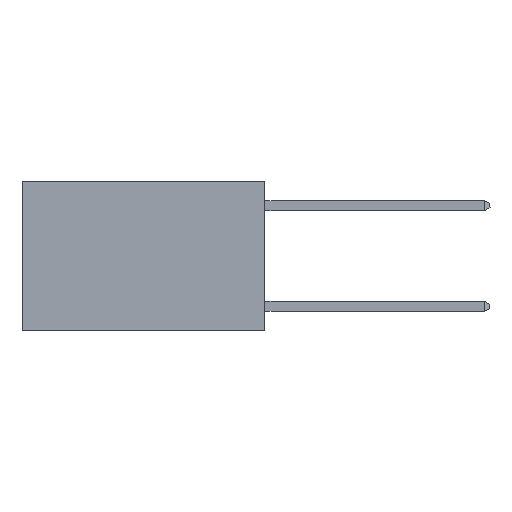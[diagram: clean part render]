
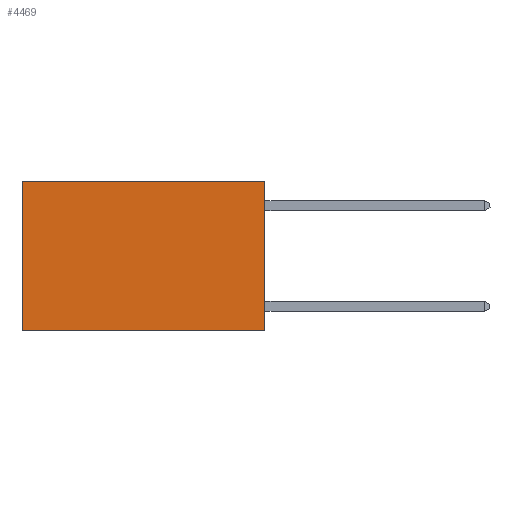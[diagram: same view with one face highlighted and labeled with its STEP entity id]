
A CAD part, left-side view. The second image highlights one B-rep face of the part: STEP entity #4469.
In plain terms, the highlighted planar face has unit normal (-1, 0, 0).
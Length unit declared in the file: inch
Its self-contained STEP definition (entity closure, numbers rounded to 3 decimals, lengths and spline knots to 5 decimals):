
#91 = FACE_OUTER_BOUND ( 'NONE', #1122, .T. ) ;
#298 = CARTESIAN_POINT ( 'NONE',  ( 0.2625, 0., 0. ) ) ;
#379 = EDGE_CURVE ( 'NONE', #6672, #7681, #6910, .T. ) ;
#523 = LINE ( 'NONE', #5374, #2490 ) ;
#844 = CARTESIAN_POINT ( 'NONE',  ( 0.2625, 0.6, -0.37 ) ) ;
#884 = PLANE ( 'NONE',  #6083 ) ;
#1122 = EDGE_LOOP ( 'NONE', ( #5897, #5910, #5946, #6079 ) ) ;
#1266 = VECTOR ( 'NONE', #5810, 39.37008 ) ;
#1371 = VECTOR ( 'NONE', #7424, 39.37008 ) ;
#1379 = CARTESIAN_POINT ( 'NONE',  ( 0.2625, 0., 0. ) ) ;
#1388 = EDGE_CURVE ( 'NONE', #7681, #3442, #1503, .T. ) ;
#1503 = LINE ( 'NONE', #5966, #1266 ) ;
#1580 = LINE ( 'NONE', #6878, #1371 ) ;
#1620 = DIRECTION ( 'NONE',  ( 1., 0., 0. ) ) ;
#1809 = VERTEX_POINT ( 'NONE', #6113 ) ;
#2490 = VECTOR ( 'NONE', #5948, 39.37008 ) ;
#3271 = DIRECTION ( 'NONE',  ( 0., 0., -1. ) ) ;
#3442 = VERTEX_POINT ( 'NONE', #844 ) ;
#3760 = CARTESIAN_POINT ( 'NONE',  ( 0.2625, 0., -0.37 ) ) ;
#3843 = EDGE_CURVE ( 'NONE', #1809, #3442, #1580, .T. ) ;
#4469 = ADVANCED_FACE ( 'NONE', ( #91 ), #884, .F. ) ;
#4678 = EDGE_CURVE ( 'NONE', #6672, #1809, #523, .T. ) ;
#5374 = CARTESIAN_POINT ( 'NONE',  ( 0.2625, 0., 0. ) ) ;
#5434 = VECTOR ( 'NONE', #3271, 39.37008 ) ;
#5810 = DIRECTION ( 'NONE',  ( 0., 1., 0. ) ) ;
#5897 = ORIENTED_EDGE ( 'NONE', *, *, #3843, .T. ) ;
#5910 = ORIENTED_EDGE ( 'NONE', *, *, #1388, .F. ) ;
#5946 = ORIENTED_EDGE ( 'NONE', *, *, #379, .F. ) ;
#5948 = DIRECTION ( 'NONE',  ( 0., 1., 0. ) ) ;
#5966 = CARTESIAN_POINT ( 'NONE',  ( 0.2625, 0., -0.37 ) ) ;
#6079 = ORIENTED_EDGE ( 'NONE', *, *, #4678, .T. ) ;
#6083 = AXIS2_PLACEMENT_3D ( 'NONE', #8147, #1620, #6566 ) ;
#6113 = CARTESIAN_POINT ( 'NONE',  ( 0.2625, 0.6, 0. ) ) ;
#6566 = DIRECTION ( 'NONE',  ( 0., 0., -1. ) ) ;
#6672 = VERTEX_POINT ( 'NONE', #1379 ) ;
#6878 = CARTESIAN_POINT ( 'NONE',  ( 0.2625, 0.6, 0. ) ) ;
#6910 = LINE ( 'NONE', #298, #5434 ) ;
#7424 = DIRECTION ( 'NONE',  ( 0., 0., -1. ) ) ;
#7681 = VERTEX_POINT ( 'NONE', #3760 ) ;
#8147 = CARTESIAN_POINT ( 'NONE',  ( 0.2625, 0., 0. ) ) ;
